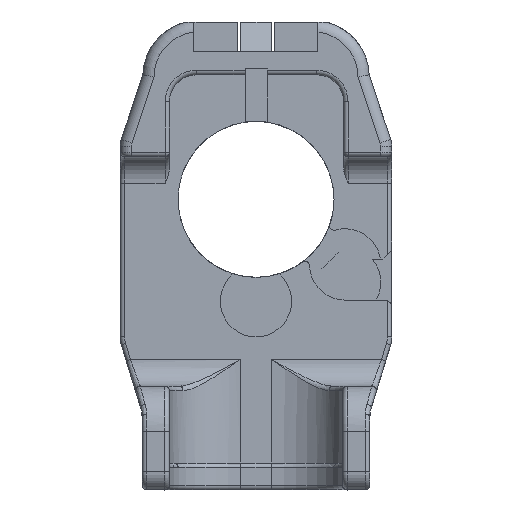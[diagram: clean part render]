
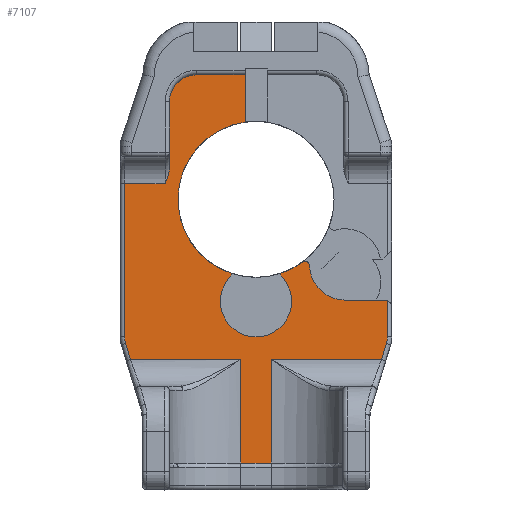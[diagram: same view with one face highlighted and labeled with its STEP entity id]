
A CAD part, front view. The second image highlights one B-rep face of the part: STEP entity #7107.
In plain terms, the highlighted planar face has unit normal (0, -1, 0).
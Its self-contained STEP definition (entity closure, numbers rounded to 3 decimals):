
#276=PLANE('',#7779);
#618=FACE_OUTER_BOUND('',#1019,.T.);
#1019=EDGE_LOOP('',(#6137,#6138,#6139,#6140,#6141,#6142,#6143,#6144,#6145,
#6146,#6147,#6148,#6149,#6150,#6151,#6152,#6153,#6154,#6155,#6156,#6157,
#6158,#6159));
#1216=CIRCLE('',#7590,2.5);
#1234=CIRCLE('',#7623,2.5);
#1296=CIRCLE('',#7745,4.);
#1309=CIRCLE('',#7762,4.);
#1310=CIRCLE('',#7769,0.5);
#1311=CIRCLE('',#7780,3.);
#1312=CIRCLE('',#7781,8.75);
#1313=CIRCLE('',#7782,8.75);
#1429=B_SPLINE_CURVE_WITH_KNOTS('',3,(#12388,#12389,#12390,#12391),
 .UNSPECIFIED.,.F.,.F.,(4,4),(0.382,0.56),
 .UNSPECIFIED.);
#1705=LINE('',#11102,#2281);
#1885=LINE('',#12318,#2461);
#1886=LINE('',#12331,#2462);
#1895=LINE('',#12409,#2471);
#1896=LINE('',#12418,#2472);
#1919=LINE('',#12549,#2495);
#1929=LINE('',#12641,#2505);
#1931=LINE('',#12651,#2507);
#1941=LINE('',#12738,#2517);
#1944=LINE('',#12742,#2520);
#1971=LINE('',#12904,#2547);
#1972=LINE('',#12908,#2548);
#1983=LINE('',#12950,#2559);
#1984=LINE('',#12956,#2560);
#2281=VECTOR('',#8476,10.);
#2461=VECTOR('',#9010,10.);
#2462=VECTOR('',#9025,10.);
#2471=VECTOR('',#9086,10.);
#2472=VECTOR('',#9099,10.);
#2495=VECTOR('',#9194,10.);
#2505=VECTOR('',#9248,10.);
#2507=VECTOR('',#9256,10.);
#2517=VECTOR('',#9314,10.);
#2520=VECTOR('',#9319,10.);
#2547=VECTOR('',#9452,10.);
#2548=VECTOR('',#9457,10.);
#2559=VECTOR('',#9492,10.);
#2560=VECTOR('',#9501,10.);
#3035=VERTEX_POINT('',#11099);
#3036=VERTEX_POINT('',#11101);
#3239=VERTEX_POINT('',#12315);
#3240=VERTEX_POINT('',#12317);
#3242=VERTEX_POINT('',#12322);
#3243=VERTEX_POINT('',#12324);
#3245=VERTEX_POINT('',#12330);
#3252=VERTEX_POINT('',#12387);
#3254=VERTEX_POINT('',#12407);
#3255=VERTEX_POINT('',#12412);
#3256=VERTEX_POINT('',#12416);
#3279=VERTEX_POINT('',#12539);
#3292=VERTEX_POINT('',#12631);
#3296=VERTEX_POINT('',#12648);
#3297=VERTEX_POINT('',#12650);
#3331=VERTEX_POINT('',#12855);
#3332=VERTEX_POINT('',#12857);
#3344=VERTEX_POINT('',#12890);
#3345=VERTEX_POINT('',#12892);
#3348=VERTEX_POINT('',#12902);
#3350=VERTEX_POINT('',#12913);
#3356=VERTEX_POINT('',#12948);
#3357=VERTEX_POINT('',#12952);
#3825=EDGE_CURVE('',#3035,#3036,#1705,.T.);
#4140=EDGE_CURVE('',#3239,#3240,#1885,.T.);
#4143=EDGE_CURVE('',#3242,#3243,#1216,.T.);
#4146=EDGE_CURVE('',#3243,#3245,#1886,.T.);
#4161=EDGE_CURVE('',#3240,#3252,#1429,.F.);
#4171=EDGE_CURVE('',#3254,#3239,#1895,.T.);
#4174=EDGE_CURVE('',#3255,#3254,#1234,.T.);
#4176=EDGE_CURVE('',#3256,#3255,#1896,.T.);
#4219=EDGE_CURVE('',#3256,#3279,#1919,.T.);
#4243=EDGE_CURVE('',#3292,#3245,#1929,.T.);
#4247=EDGE_CURVE('',#3297,#3296,#1931,.T.);
#4272=EDGE_CURVE('',#3297,#3279,#1941,.T.);
#4275=EDGE_CURVE('',#3292,#3296,#1944,.T.);
#4312=EDGE_CURVE('',#3332,#3331,#1296,.T.);
#4330=EDGE_CURVE('',#3345,#3344,#1309,.T.);
#4336=EDGE_CURVE('',#3345,#3348,#1971,.T.);
#4338=EDGE_CURVE('',#3348,#3242,#1972,.T.);
#4341=EDGE_CURVE('',#3350,#3344,#1310,.T.);
#4355=EDGE_CURVE('',#3356,#3252,#1983,.T.);
#4356=EDGE_CURVE('',#3357,#3356,#1311,.T.);
#4357=EDGE_CURVE('',#3350,#3332,#1312,.T.);
#4358=EDGE_CURVE('',#3331,#3036,#1313,.T.);
#4359=EDGE_CURVE('',#3035,#3357,#1984,.T.);
#6137=ORIENTED_EDGE('',*,*,#4356,.T.);
#6138=ORIENTED_EDGE('',*,*,#4355,.T.);
#6139=ORIENTED_EDGE('',*,*,#4161,.F.);
#6140=ORIENTED_EDGE('',*,*,#4140,.F.);
#6141=ORIENTED_EDGE('',*,*,#4171,.F.);
#6142=ORIENTED_EDGE('',*,*,#4174,.F.);
#6143=ORIENTED_EDGE('',*,*,#4176,.F.);
#6144=ORIENTED_EDGE('',*,*,#4219,.T.);
#6145=ORIENTED_EDGE('',*,*,#4272,.F.);
#6146=ORIENTED_EDGE('',*,*,#4247,.T.);
#6147=ORIENTED_EDGE('',*,*,#4275,.F.);
#6148=ORIENTED_EDGE('',*,*,#4243,.T.);
#6149=ORIENTED_EDGE('',*,*,#4146,.F.);
#6150=ORIENTED_EDGE('',*,*,#4143,.F.);
#6151=ORIENTED_EDGE('',*,*,#4338,.F.);
#6152=ORIENTED_EDGE('',*,*,#4336,.F.);
#6153=ORIENTED_EDGE('',*,*,#4330,.T.);
#6154=ORIENTED_EDGE('',*,*,#4341,.F.);
#6155=ORIENTED_EDGE('',*,*,#4357,.T.);
#6156=ORIENTED_EDGE('',*,*,#4312,.T.);
#6157=ORIENTED_EDGE('',*,*,#4358,.T.);
#6158=ORIENTED_EDGE('',*,*,#3825,.F.);
#6159=ORIENTED_EDGE('',*,*,#4359,.T.);
#7107=ADVANCED_FACE('',(#618),#276,.T.);
#7590=AXIS2_PLACEMENT_3D('',#12325,#9017,#9018);
#7623=AXIS2_PLACEMENT_3D('',#12414,#9093,#9094);
#7745=AXIS2_PLACEMENT_3D('',#12858,#9402,#9403);
#7762=AXIS2_PLACEMENT_3D('',#12893,#9441,#9442);
#7769=AXIS2_PLACEMENT_3D('',#12914,#9464,#9465);
#7779=AXIS2_PLACEMENT_3D('',#12951,#9493,#9494);
#7780=AXIS2_PLACEMENT_3D('',#12953,#9495,#9496);
#7781=AXIS2_PLACEMENT_3D('',#12954,#9497,#9498);
#7782=AXIS2_PLACEMENT_3D('',#12955,#9499,#9500);
#8476=DIRECTION('',(0.,0.,-1.));
#9010=DIRECTION('',(1.,0.,0.));
#9017=DIRECTION('center_axis',(0.,1.,0.));
#9018=DIRECTION('ref_axis',(0.989,0.,-0.149));
#9025=DIRECTION('',(-0.294,0.,-0.956));
#9086=DIRECTION('',(0.,0.,1.));
#9093=DIRECTION('center_axis',(0.,1.,0.));
#9094=DIRECTION('ref_axis',(-0.989,0.,-0.149));
#9099=DIRECTION('',(-0.294,0.,0.956));
#9194=DIRECTION('',(1.,0.,0.));
#9248=DIRECTION('',(1.,0.,0.));
#9256=DIRECTION('',(1.,0.,0.));
#9314=DIRECTION('',(0.,0.,1.));
#9319=DIRECTION('',(0.,0.,-1.));
#9402=DIRECTION('center_axis',(0.,1.,0.));
#9403=DIRECTION('ref_axis',(1.,0.,0.));
#9441=DIRECTION('center_axis',(0.,1.,0.));
#9442=DIRECTION('ref_axis',(-0.751,0.,0.66));
#9452=DIRECTION('',(1.,0.,0.));
#9457=DIRECTION('',(0.,0.,-1.));
#9464=DIRECTION('center_axis',(0.,1.,0.));
#9465=DIRECTION('ref_axis',(0.437,0.,0.9));
#9492=DIRECTION('',(0.,0.,-1.));
#9493=DIRECTION('center_axis',(0.,-1.,0.));
#9494=DIRECTION('ref_axis',(0.,0.,-1.));
#9495=DIRECTION('center_axis',(0.,-1.,0.));
#9496=DIRECTION('ref_axis',(-1.,0.,0.));
#9497=DIRECTION('center_axis',(0.,1.,0.));
#9498=DIRECTION('ref_axis',(-1.,0.,0.));
#9499=DIRECTION('center_axis',(0.,1.,0.));
#9500=DIRECTION('ref_axis',(-1.,0.,0.));
#9501=DIRECTION('',(-1.,0.,0.));
#11099=CARTESIAN_POINT('',(-1.212,65.024,-279.606));
#11101=CARTESIAN_POINT('',(-1.212,65.024,-284.904));
#11102=CARTESIAN_POINT('',(-1.212,65.024,-291.281));
#12315=CARTESIAN_POINT('',(-14.74,65.024,-291.805));
#12317=CARTESIAN_POINT('',(-10.192,65.024,-291.805));
#12318=CARTESIAN_POINT('',(-13.97,65.024,-291.805));
#12322=CARTESIAN_POINT('',(14.74,65.024,-308.994));
#12324=CARTESIAN_POINT('',(14.629,65.024,-309.729));
#12325=CARTESIAN_POINT('Origin',(12.24,65.024,-308.994));
#12330=CARTESIAN_POINT('',(14.077,65.024,-311.525));
#12331=CARTESIAN_POINT('',(16.519,65.024,-303.587));
#12387=CARTESIAN_POINT('',(-9.692,65.024,-290.002));
#12388=CARTESIAN_POINT('Ctrl Pts',(-9.692,65.024,-290.002));
#12389=CARTESIAN_POINT('Ctrl Pts',(-9.692,65.024,-290.597));
#12390=CARTESIAN_POINT('Ctrl Pts',(-9.968,65.024,-291.255));
#12391=CARTESIAN_POINT('Ctrl Pts',(-10.192,65.024,-291.805));
#12407=CARTESIAN_POINT('',(-14.74,65.024,-308.994));
#12409=CARTESIAN_POINT('',(-14.74,65.024,-295.95));
#12412=CARTESIAN_POINT('',(-14.629,65.024,-309.729));
#12414=CARTESIAN_POINT('Origin',(-12.24,65.024,-308.994));
#12416=CARTESIAN_POINT('',(-14.077,65.024,-311.525));
#12418=CARTESIAN_POINT('',(-15.078,65.024,-308.272));
#12539=CARTESIAN_POINT('',(-1.723,65.024,-311.525));
#12549=CARTESIAN_POINT('',(-10.795,65.024,-311.525));
#12631=CARTESIAN_POINT('',(1.723,65.024,-311.525));
#12641=CARTESIAN_POINT('',(1.27,65.024,-311.525));
#12648=CARTESIAN_POINT('',(1.723,65.024,-323.145));
#12650=CARTESIAN_POINT('',(-1.723,65.024,-323.145));
#12651=CARTESIAN_POINT('',(-6.35,65.024,-323.145));
#12738=CARTESIAN_POINT('',(-1.723,65.024,-313.763));
#12742=CARTESIAN_POINT('',(1.723,65.024,-306.066));
#12855=CARTESIAN_POINT('',(-2.569,65.024,-301.934));
#12857=CARTESIAN_POINT('',(2.569,65.024,-301.934));
#12858=CARTESIAN_POINT('Origin',(0.,65.024,-305.));
#12890=CARTESIAN_POINT('',(6.002,65.024,-300.991));
#12892=CARTESIAN_POINT('',(9.906,65.024,-304.871));
#12893=CARTESIAN_POINT('Origin',(10.,65.024,-300.872));
#12902=CARTESIAN_POINT('',(14.74,65.024,-304.871));
#12904=CARTESIAN_POINT('',(9.953,65.024,-304.871));
#12908=CARTESIAN_POINT('',(14.74,65.024,-295.945));
#12913=CARTESIAN_POINT('',(5.205,65.024,-300.604));
#12914=CARTESIAN_POINT('Origin',(5.502,65.024,-301.006));
#12948=CARTESIAN_POINT('',(-9.692,65.024,-282.606));
#12950=CARTESIAN_POINT('',(-9.692,65.024,-293.093));
#12951=CARTESIAN_POINT('Origin',(-12.7,65.024,-297.382));
#12952=CARTESIAN_POINT('',(-6.692,65.024,-279.606));
#12953=CARTESIAN_POINT('Origin',(-6.692,65.024,-282.606));
#12954=CARTESIAN_POINT('Origin',(0.,65.024,-293.57));
#12955=CARTESIAN_POINT('Origin',(0.,65.024,-293.57));
#12956=CARTESIAN_POINT('',(-12.701,65.024,-279.606));
